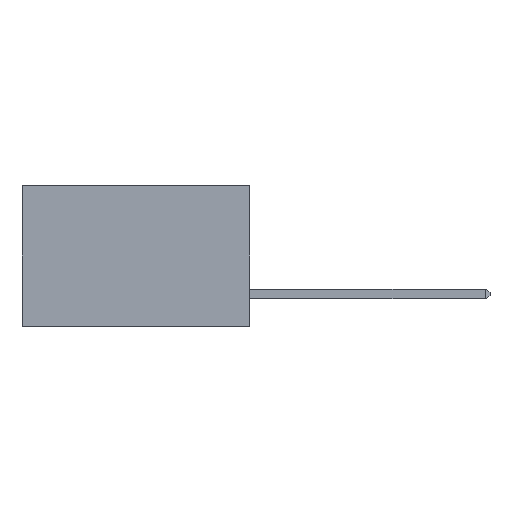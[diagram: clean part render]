
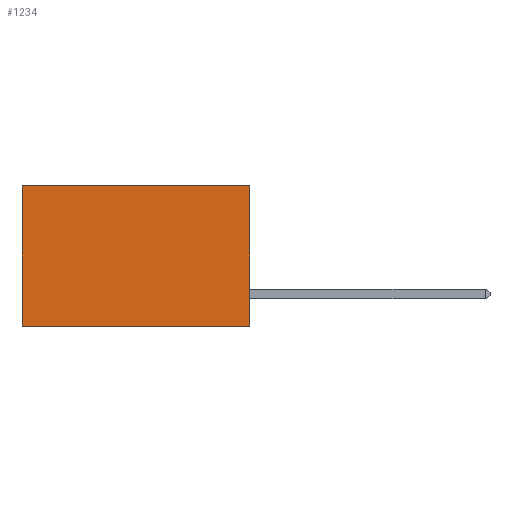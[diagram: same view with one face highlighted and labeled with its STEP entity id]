
A CAD part, left-side view. The second image highlights one B-rep face of the part: STEP entity #1234.
In plain terms, the highlighted planar face has unit normal (-1, 0, 0).
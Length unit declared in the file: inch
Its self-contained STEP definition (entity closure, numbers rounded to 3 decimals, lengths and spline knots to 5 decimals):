
#110 = EDGE_CURVE ( 'NONE', #701, #3798, #982, .T. ) ;
#156 = VERTEX_POINT ( 'NONE', #193 ) ;
#193 = CARTESIAN_POINT ( 'NONE',  ( 0.2875, 0., -0.37 ) ) ;
#701 = VERTEX_POINT ( 'NONE', #4065 ) ;
#982 = LINE ( 'NONE', #6025, #3206 ) ;
#1234 = ADVANCED_FACE ( 'NONE', ( #4487 ), #7000, .F. ) ;
#1339 = CARTESIAN_POINT ( 'NONE',  ( 0.2875, 0.6, 0. ) ) ;
#2283 = VECTOR ( 'NONE', #4048, 39.37008 ) ;
#2370 = ORIENTED_EDGE ( 'NONE', *, *, #110, .T. ) ;
#2391 = CARTESIAN_POINT ( 'NONE',  ( 0.2875, 0., 0. ) ) ;
#3206 = VECTOR ( 'NONE', #3890, 39.37008 ) ;
#3209 = CARTESIAN_POINT ( 'NONE',  ( 0.2875, 0.6, 0. ) ) ;
#3798 = VERTEX_POINT ( 'NONE', #1339 ) ;
#3890 = DIRECTION ( 'NONE',  ( 0., 1., 0. ) ) ;
#3928 = LINE ( 'NONE', #6728, #4462 ) ;
#4048 = DIRECTION ( 'NONE',  ( 0., 0., -1. ) ) ;
#4054 = EDGE_CURVE ( 'NONE', #156, #8513, #3928, .T. ) ;
#4065 = CARTESIAN_POINT ( 'NONE',  ( 0.2875, 0., 0. ) ) ;
#4462 = VECTOR ( 'NONE', #6719, 39.37008 ) ;
#4487 = FACE_OUTER_BOUND ( 'NONE', #9798, .T. ) ;
#4507 = CARTESIAN_POINT ( 'NONE',  ( 0.2875, 0., 0. ) ) ;
#4515 = AXIS2_PLACEMENT_3D ( 'NONE', #2391, #4680, #4679 ) ;
#4679 = DIRECTION ( 'NONE',  ( 0., 0., -1. ) ) ;
#4680 = DIRECTION ( 'NONE',  ( 1., 0., 0. ) ) ;
#4687 = ORIENTED_EDGE ( 'NONE', *, *, #9065, .F. ) ;
#6025 = CARTESIAN_POINT ( 'NONE',  ( 0.2875, 0., 0. ) ) ;
#6684 = ORIENTED_EDGE ( 'NONE', *, *, #4054, .F. ) ;
#6719 = DIRECTION ( 'NONE',  ( 0., 1., 0. ) ) ;
#6728 = CARTESIAN_POINT ( 'NONE',  ( 0.2875, 0., -0.37 ) ) ;
#6856 = LINE ( 'NONE', #3209, #2283 ) ;
#7000 = PLANE ( 'NONE',  #4515 ) ;
#7260 = CARTESIAN_POINT ( 'NONE',  ( 0.2875, 0.6, -0.37 ) ) ;
#8074 = LINE ( 'NONE', #4507, #9880 ) ;
#8513 = VERTEX_POINT ( 'NONE', #7260 ) ;
#9065 = EDGE_CURVE ( 'NONE', #701, #156, #8074, .T. ) ;
#9798 = EDGE_LOOP ( 'NONE', ( #10505, #6684, #4687, #2370 ) ) ;
#9880 = VECTOR ( 'NONE', #10857, 39.37008 ) ;
#10029 = EDGE_CURVE ( 'NONE', #3798, #8513, #6856, .T. ) ;
#10505 = ORIENTED_EDGE ( 'NONE', *, *, #10029, .T. ) ;
#10857 = DIRECTION ( 'NONE',  ( 0., 0., -1. ) ) ;
